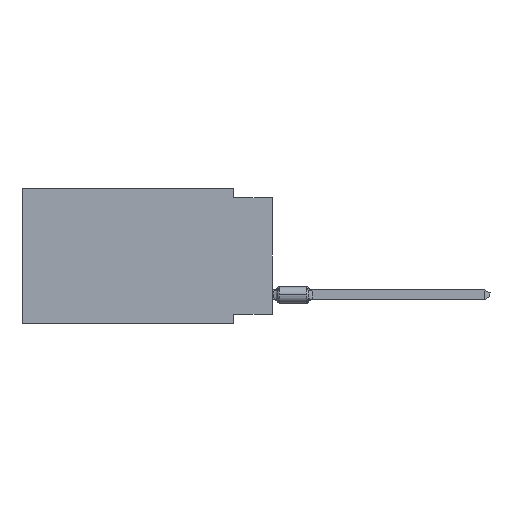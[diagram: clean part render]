
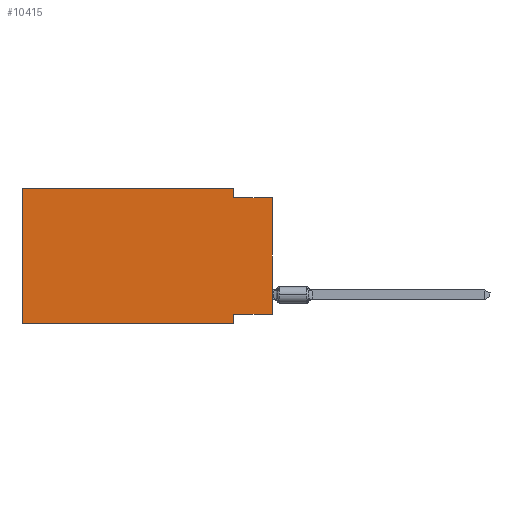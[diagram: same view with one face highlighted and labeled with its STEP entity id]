
A CAD part, left-side view. The second image highlights one B-rep face of the part: STEP entity #10415.
In plain terms, the highlighted planar face has unit normal (-1, 0, 0).
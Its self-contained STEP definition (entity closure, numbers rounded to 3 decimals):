
#515 = LINE ( 'NONE', #7828, #15696 ) ;
#1305 = ORIENTED_EDGE ( 'NONE', *, *, #40198, .T. ) ;
#1345 = VECTOR ( 'NONE', #34275, 1000. ) ;
#2178 = ORIENTED_EDGE ( 'NONE', *, *, #14212, .F. ) ;
#2992 = CARTESIAN_POINT ( 'NONE',  ( 0., 2.54, -8.255 ) ) ;
#3388 = VECTOR ( 'NONE', #6307, 1000. ) ;
#3951 = VECTOR ( 'NONE', #7229, 1000. ) ;
#4405 = CARTESIAN_POINT ( 'NONE',  ( 0., 16.383, -8.89 ) ) ;
#4815 = CARTESIAN_POINT ( 'NONE',  ( 0., 16.383, -8.89 ) ) ;
#5057 = LINE ( 'NONE', #37548, #35603 ) ;
#5952 = VERTEX_POINT ( 'NONE', #20646 ) ;
#6307 = DIRECTION ( 'NONE',  ( 0., 0., -1. ) ) ;
#6576 = EDGE_CURVE ( 'NONE', #29248, #22827, #28452, .T. ) ;
#6984 = CARTESIAN_POINT ( 'NONE',  ( 0., 16.383, 0. ) ) ;
#7229 = DIRECTION ( 'NONE',  ( 0., 0., -1. ) ) ;
#7828 = CARTESIAN_POINT ( 'NONE',  ( 0., 0., 0. ) ) ;
#8085 = ORIENTED_EDGE ( 'NONE', *, *, #20700, .F. ) ;
#9919 = LINE ( 'NONE', #43542, #3951 ) ;
#10415 = ADVANCED_FACE ( 'NONE', ( #38346 ), #38574, .F. ) ;
#10496 = ORIENTED_EDGE ( 'NONE', *, *, #26458, .T. ) ;
#12100 = VERTEX_POINT ( 'NONE', #2992 ) ;
#14075 = CARTESIAN_POINT ( 'NONE',  ( 0., 2.54, 0. ) ) ;
#14212 = EDGE_CURVE ( 'NONE', #12100, #46405, #9919, .T. ) ;
#15696 = VECTOR ( 'NONE', #45087, 1000. ) ;
#16065 = AXIS2_PLACEMENT_3D ( 'NONE', #41985, #31016, #35174 ) ;
#17121 = ORIENTED_EDGE ( 'NONE', *, *, #24575, .F. ) ;
#19586 = DIRECTION ( 'NONE',  ( 0., -1., 0. ) ) ;
#20646 = CARTESIAN_POINT ( 'NONE',  ( 0., 0., -0.635 ) ) ;
#20700 = EDGE_CURVE ( 'NONE', #41833, #29248, #43729, .T. ) ;
#22827 = VERTEX_POINT ( 'NONE', #28150 ) ;
#24575 = EDGE_CURVE ( 'NONE', #47101, #41833, #46109, .T. ) ;
#25019 = VERTEX_POINT ( 'NONE', #35567 ) ;
#25598 = EDGE_CURVE ( 'NONE', #22827, #5952, #5057, .T. ) ;
#26458 = EDGE_CURVE ( 'NONE', #25019, #5952, #515, .T. ) ;
#27665 = LINE ( 'NONE', #4815, #1345 ) ;
#27877 = CARTESIAN_POINT ( 'NONE',  ( 0., 2.54, -8.89 ) ) ;
#28150 = CARTESIAN_POINT ( 'NONE',  ( 0., 2.54, -0.635 ) ) ;
#28381 = ORIENTED_EDGE ( 'NONE', *, *, #6576, .F. ) ;
#28452 = LINE ( 'NONE', #14075, #3388 ) ;
#29248 = VERTEX_POINT ( 'NONE', #44426 ) ;
#29579 = VECTOR ( 'NONE', #19586, 1000. ) ;
#29616 = CARTESIAN_POINT ( 'NONE',  ( 0., 0., -8.255 ) ) ;
#30327 = DIRECTION ( 'NONE',  ( 0., 1., 0. ) ) ;
#31016 = DIRECTION ( 'NONE',  ( 1., 0., 0. ) ) ;
#31245 = DIRECTION ( 'NONE',  ( 0., 0., 1. ) ) ;
#32589 = EDGE_CURVE ( 'NONE', #25019, #12100, #48118, .T. ) ;
#33528 = ORIENTED_EDGE ( 'NONE', *, *, #25598, .F. ) ;
#34275 = DIRECTION ( 'NONE',  ( 0., -1., 0. ) ) ;
#34442 = CARTESIAN_POINT ( 'NONE',  ( 0., 16.383, 0. ) ) ;
#35174 = DIRECTION ( 'NONE',  ( 0., 0., -1. ) ) ;
#35567 = CARTESIAN_POINT ( 'NONE',  ( 0., 0., -8.255 ) ) ;
#35603 = VECTOR ( 'NONE', #38926, 1000. ) ;
#37548 = CARTESIAN_POINT ( 'NONE',  ( 0., 0., -0.635 ) ) ;
#38346 = FACE_OUTER_BOUND ( 'NONE', #39744, .T. ) ;
#38574 = PLANE ( 'NONE',  #16065 ) ;
#38926 = DIRECTION ( 'NONE',  ( 0., -1., 0. ) ) ;
#39026 = VECTOR ( 'NONE', #31245, 1000. ) ;
#39744 = EDGE_LOOP ( 'NONE', ( #10496, #33528, #28381, #8085, #17121, #1305, #2178, #48122 ) ) ;
#39971 = VECTOR ( 'NONE', #30327, 1000. ) ;
#40198 = EDGE_CURVE ( 'NONE', #47101, #46405, #27665, .T. ) ;
#41833 = VERTEX_POINT ( 'NONE', #6984 ) ;
#41985 = CARTESIAN_POINT ( 'NONE',  ( 0., 16.383, 0. ) ) ;
#43542 = CARTESIAN_POINT ( 'NONE',  ( 0., 2.54, -8.89 ) ) ;
#43729 = LINE ( 'NONE', #34442, #29579 ) ;
#44426 = CARTESIAN_POINT ( 'NONE',  ( 0., 2.54, 0. ) ) ;
#45087 = DIRECTION ( 'NONE',  ( 0., 0., 1. ) ) ;
#45390 = CARTESIAN_POINT ( 'NONE',  ( 0., 16.383, 0. ) ) ;
#46109 = LINE ( 'NONE', #45390, #39026 ) ;
#46405 = VERTEX_POINT ( 'NONE', #27877 ) ;
#47101 = VERTEX_POINT ( 'NONE', #4405 ) ;
#48118 = LINE ( 'NONE', #29616, #39971 ) ;
#48122 = ORIENTED_EDGE ( 'NONE', *, *, #32589, .F. ) ;
